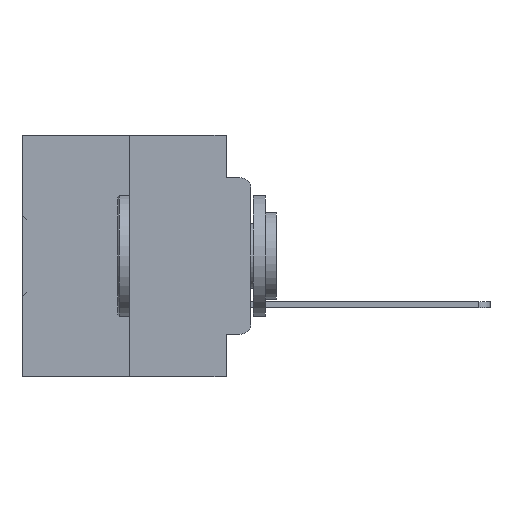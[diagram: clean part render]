
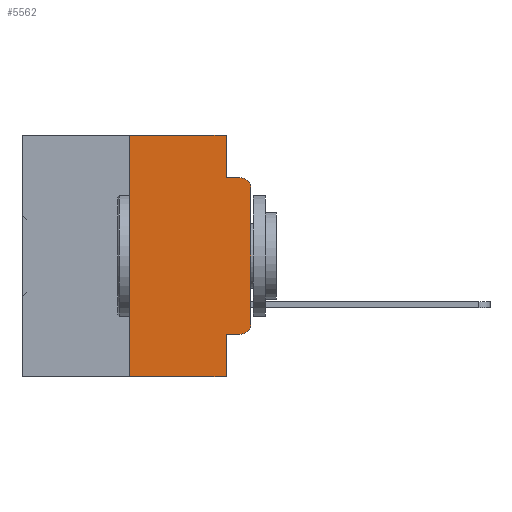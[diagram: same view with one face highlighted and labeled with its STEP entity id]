
A CAD part, left-side view. The second image highlights one B-rep face of the part: STEP entity #5562.
In plain terms, the highlighted planar face has unit normal (-1, 0, 0).
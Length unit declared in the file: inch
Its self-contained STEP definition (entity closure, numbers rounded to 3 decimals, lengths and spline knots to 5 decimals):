
#212 = LINE ( 'NONE', #1967, #21001 ) ;
#238 = CARTESIAN_POINT ( 'NONE',  ( 0., 0.473, 0. ) ) ;
#365 = LINE ( 'NONE', #16851, #6428 ) ;
#1141 = VERTEX_POINT ( 'NONE', #11413 ) ;
#1967 = CARTESIAN_POINT ( 'NONE',  ( 0., 0.051, -0.4115 ) ) ;
#3213 = PLANE ( 'NONE',  #8147 ) ;
#4315 = CARTESIAN_POINT ( 'NONE',  ( 0., 0.25, 0. ) ) ;
#4725 = VERTEX_POINT ( 'NONE', #30403 ) ;
#5291 = EDGE_CURVE ( 'NONE', #13263, #31354, #365, .T. ) ;
#5436 = ORIENTED_EDGE ( 'NONE', *, *, #33433, .T. ) ;
#5562 = ADVANCED_FACE ( 'NONE', ( #29313 ), #3213, .F. ) ;
#6132 = CARTESIAN_POINT ( 'NONE',  ( 0., 0., 0. ) ) ;
#6239 = DIRECTION ( 'NONE',  ( 0., 0., -1. ) ) ;
#6428 = VECTOR ( 'NONE', #10946, 39.37008 ) ;
#6853 = CARTESIAN_POINT ( 'NONE',  ( 0., 0.473, 0. ) ) ;
#7240 = DIRECTION ( 'NONE',  ( -1., 0., 0. ) ) ;
#7340 = EDGE_CURVE ( 'NONE', #4725, #1141, #30923, .T. ) ;
#7634 = VECTOR ( 'NONE', #8177, 39.37008 ) ;
#7693 = CARTESIAN_POINT ( 'NONE',  ( 0., 0.051, -0.4115 ) ) ;
#8065 = LINE ( 'NONE', #28367, #22734 ) ;
#8147 = AXIS2_PLACEMENT_3D ( 'NONE', #238, #15057, #6239 ) ;
#8177 = DIRECTION ( 'NONE',  ( 0., 0., -1. ) ) ;
#9342 = EDGE_CURVE ( 'NONE', #1141, #9532, #26546, .T. ) ;
#9532 = VERTEX_POINT ( 'NONE', #18275 ) ;
#9860 = DIRECTION ( 'NONE',  ( 0., -1., 0. ) ) ;
#10030 = LINE ( 'NONE', #6853, #24651 ) ;
#10946 = DIRECTION ( 'NONE',  ( 0., 0., 1. ) ) ;
#11413 = CARTESIAN_POINT ( 'NONE',  ( 0., 0.051, -0.0885 ) ) ;
#11501 = ORIENTED_EDGE ( 'NONE', *, *, #35320, .F. ) ;
#11790 = EDGE_LOOP ( 'NONE', ( #24740, #18805, #20630, #36834, #15644, #16562, #26119, #11501, #5436, #16514 ) ) ;
#11861 = CARTESIAN_POINT ( 'NONE',  ( 0., 0.02, -0.3915 ) ) ;
#12591 = LINE ( 'NONE', #6132, #33904 ) ;
#13224 = CARTESIAN_POINT ( 'NONE',  ( 0., 0., -0.3915 ) ) ;
#13263 = VERTEX_POINT ( 'NONE', #22454 ) ;
#14057 = EDGE_CURVE ( 'NONE', #31354, #4725, #10030, .T. ) ;
#14828 = DIRECTION ( 'NONE',  ( 0., 0., -1. ) ) ;
#15057 = DIRECTION ( 'NONE',  ( 1., 0., 0. ) ) ;
#15085 = DIRECTION ( 'NONE',  ( 0., 0., 1. ) ) ;
#15644 = ORIENTED_EDGE ( 'NONE', *, *, #14057, .F. ) ;
#16514 = ORIENTED_EDGE ( 'NONE', *, *, #31523, .T. ) ;
#16562 = ORIENTED_EDGE ( 'NONE', *, *, #5291, .F. ) ;
#16851 = CARTESIAN_POINT ( 'NONE',  ( 0., 0.25, 0. ) ) ;
#16921 = CARTESIAN_POINT ( 'NONE',  ( 0., 0.051, 0. ) ) ;
#17193 = EDGE_CURVE ( 'NONE', #33241, #9532, #23486, .T. ) ;
#18034 = AXIS2_PLACEMENT_3D ( 'NONE', #11861, #32191, #14828 ) ;
#18275 = CARTESIAN_POINT ( 'NONE',  ( 0., 0.02, -0.0885 ) ) ;
#18490 = VERTEX_POINT ( 'NONE', #35067 ) ;
#18627 = VERTEX_POINT ( 'NONE', #21360 ) ;
#18798 = VECTOR ( 'NONE', #25145, 39.37008 ) ;
#18805 = ORIENTED_EDGE ( 'NONE', *, *, #17193, .T. ) ;
#18872 = CIRCLE ( 'NONE', #18034, 0.02 ) ;
#19151 = EDGE_CURVE ( 'NONE', #24159, #33241, #12591, .T. ) ;
#20630 = ORIENTED_EDGE ( 'NONE', *, *, #9342, .F. ) ;
#21001 = VECTOR ( 'NONE', #34167, 39.37008 ) ;
#21048 = LINE ( 'NONE', #28028, #35455 ) ;
#21360 = CARTESIAN_POINT ( 'NONE',  ( 0., 0.02, -0.4115 ) ) ;
#21621 = EDGE_CURVE ( 'NONE', #13263, #18490, #21048, .T. ) ;
#21671 = AXIS2_PLACEMENT_3D ( 'NONE', #24793, #7240, #27708 ) ;
#22454 = CARTESIAN_POINT ( 'NONE',  ( 0., 0.25, -0.5 ) ) ;
#22734 = VECTOR ( 'NONE', #31231, 39.37008 ) ;
#23486 = CIRCLE ( 'NONE', #21671, 0.02 ) ;
#24159 = VERTEX_POINT ( 'NONE', #13224 ) ;
#24651 = VECTOR ( 'NONE', #9860, 39.37008 ) ;
#24655 = CARTESIAN_POINT ( 'NONE',  ( 0., 0., -0.1085 ) ) ;
#24740 = ORIENTED_EDGE ( 'NONE', *, *, #19151, .T. ) ;
#24793 = CARTESIAN_POINT ( 'NONE',  ( 0., 0.02, -0.1085 ) ) ;
#25145 = DIRECTION ( 'NONE',  ( 0., -1., 0. ) ) ;
#26119 = ORIENTED_EDGE ( 'NONE', *, *, #21621, .T. ) ;
#26546 = LINE ( 'NONE', #36538, #18798 ) ;
#27708 = DIRECTION ( 'NONE',  ( 0., 0., -1. ) ) ;
#28028 = CARTESIAN_POINT ( 'NONE',  ( 0., 0.473, -0.5 ) ) ;
#28367 = CARTESIAN_POINT ( 'NONE',  ( 0., 0.051, 0. ) ) ;
#29313 = FACE_OUTER_BOUND ( 'NONE', #11790, .T. ) ;
#30403 = CARTESIAN_POINT ( 'NONE',  ( 0., 0.051, 0. ) ) ;
#30911 = DIRECTION ( 'NONE',  ( 0., -1., 0. ) ) ;
#30923 = LINE ( 'NONE', #16921, #7634 ) ;
#31231 = DIRECTION ( 'NONE',  ( 0., 0., -1. ) ) ;
#31354 = VERTEX_POINT ( 'NONE', #4315 ) ;
#31523 = EDGE_CURVE ( 'NONE', #18627, #24159, #18872, .T. ) ;
#32191 = DIRECTION ( 'NONE',  ( -1., 0., 0. ) ) ;
#33241 = VERTEX_POINT ( 'NONE', #24655 ) ;
#33433 = EDGE_CURVE ( 'NONE', #36536, #18627, #212, .T. ) ;
#33904 = VECTOR ( 'NONE', #15085, 39.37008 ) ;
#34167 = DIRECTION ( 'NONE',  ( 0., -1., 0. ) ) ;
#35067 = CARTESIAN_POINT ( 'NONE',  ( 0., 0.051, -0.5 ) ) ;
#35320 = EDGE_CURVE ( 'NONE', #36536, #18490, #8065, .T. ) ;
#35455 = VECTOR ( 'NONE', #30911, 39.37008 ) ;
#36536 = VERTEX_POINT ( 'NONE', #7693 ) ;
#36538 = CARTESIAN_POINT ( 'NONE',  ( 0., 0.051, -0.0885 ) ) ;
#36834 = ORIENTED_EDGE ( 'NONE', *, *, #7340, .F. ) ;
